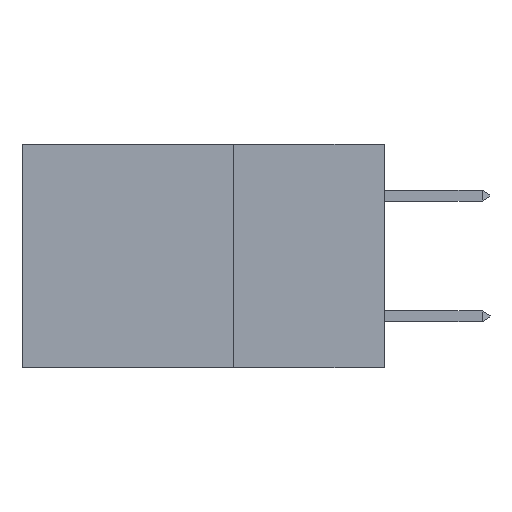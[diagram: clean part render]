
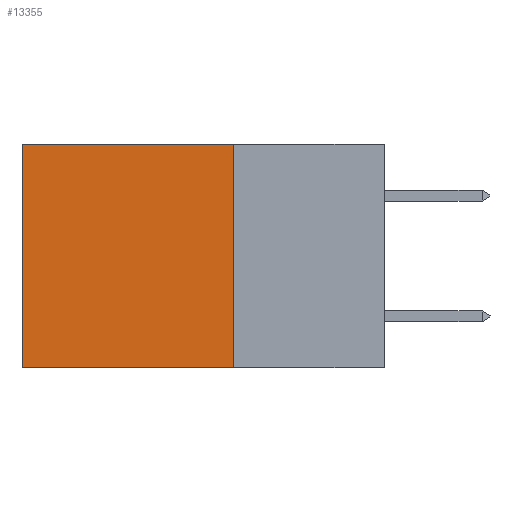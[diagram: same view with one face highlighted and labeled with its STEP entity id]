
A CAD part, left-side view. The second image highlights one B-rep face of the part: STEP entity #13355.
In plain terms, the highlighted planar face has unit normal (-1, 0, 0).
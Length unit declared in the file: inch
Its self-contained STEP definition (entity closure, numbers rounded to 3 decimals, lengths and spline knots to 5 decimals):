
#18 = FACE_OUTER_BOUND ( 'NONE', #27335, .T. ) ;
#65 = VECTOR ( 'NONE', #35724, 39.37008 ) ;
#198 = DIRECTION ( 'NONE',  ( 1., 0., 0. ) ) ;
#823 = EDGE_CURVE ( 'NONE', #23167, #28257, #32746, .T. ) ;
#2962 = LINE ( 'NONE', #6126, #20245 ) ;
#6126 = CARTESIAN_POINT ( 'NONE',  ( 0.2875, 0.25, 0. ) ) ;
#6553 = EDGE_CURVE ( 'NONE', #23167, #20212, #2962, .T. ) ;
#7940 = AXIS2_PLACEMENT_3D ( 'NONE', #11374, #198, #34266 ) ;
#8585 = DIRECTION ( 'NONE',  ( 0., 0., -1. ) ) ;
#9912 = ORIENTED_EDGE ( 'NONE', *, *, #823, .T. ) ;
#10297 = VECTOR ( 'NONE', #24534, 39.37008 ) ;
#10603 = ORIENTED_EDGE ( 'NONE', *, *, #26888, .F. ) ;
#10690 = ORIENTED_EDGE ( 'NONE', *, *, #33228, .T. ) ;
#11183 = CARTESIAN_POINT ( 'NONE',  ( 0.2875, 0.6, -0.37 ) ) ;
#11374 = CARTESIAN_POINT ( 'NONE',  ( 0.2875, 0.25, 0. ) ) ;
#13355 = ADVANCED_FACE ( 'NONE', ( #18 ), #25538, .F. ) ;
#13581 = CARTESIAN_POINT ( 'NONE',  ( 0.2875, 0.25, 0. ) ) ;
#14177 = LINE ( 'NONE', #25539, #24237 ) ;
#17317 = DIRECTION ( 'NONE',  ( 0., 0., -1. ) ) ;
#20212 = VERTEX_POINT ( 'NONE', #31994 ) ;
#20245 = VECTOR ( 'NONE', #17317, 39.37008 ) ;
#21040 = CARTESIAN_POINT ( 'NONE',  ( 0.2875, 0.25, -0.37 ) ) ;
#23167 = VERTEX_POINT ( 'NONE', #27072 ) ;
#24237 = VECTOR ( 'NONE', #8585, 39.37008 ) ;
#24534 = DIRECTION ( 'NONE',  ( 0., 1., 0. ) ) ;
#25063 = VERTEX_POINT ( 'NONE', #11183 ) ;
#25538 = PLANE ( 'NONE',  #7940 ) ;
#25539 = CARTESIAN_POINT ( 'NONE',  ( 0.2875, 0.6, 0. ) ) ;
#26888 = EDGE_CURVE ( 'NONE', #20212, #25063, #30107, .T. ) ;
#27072 = CARTESIAN_POINT ( 'NONE',  ( 0.2875, 0.25, 0. ) ) ;
#27335 = EDGE_LOOP ( 'NONE', ( #10690, #10603, #33600, #9912 ) ) ;
#28257 = VERTEX_POINT ( 'NONE', #32915 ) ;
#30107 = LINE ( 'NONE', #21040, #10297 ) ;
#31994 = CARTESIAN_POINT ( 'NONE',  ( 0.2875, 0.25, -0.37 ) ) ;
#32746 = LINE ( 'NONE', #13581, #65 ) ;
#32915 = CARTESIAN_POINT ( 'NONE',  ( 0.2875, 0.6, 0. ) ) ;
#33228 = EDGE_CURVE ( 'NONE', #28257, #25063, #14177, .T. ) ;
#33600 = ORIENTED_EDGE ( 'NONE', *, *, #6553, .F. ) ;
#34266 = DIRECTION ( 'NONE',  ( 0., 0., -1. ) ) ;
#35724 = DIRECTION ( 'NONE',  ( 0., 1., 0. ) ) ;
